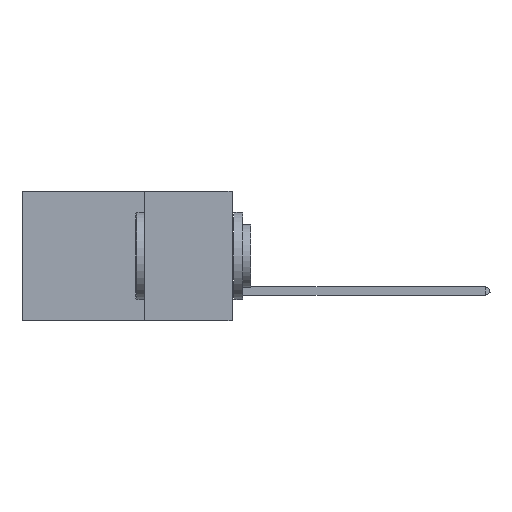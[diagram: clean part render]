
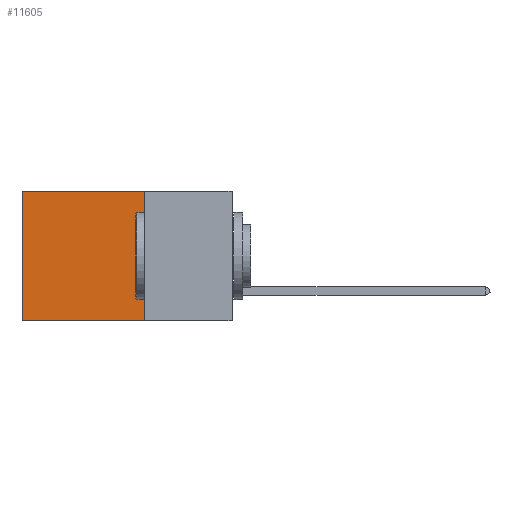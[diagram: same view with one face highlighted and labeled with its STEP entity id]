
A CAD part, left-side view. The second image highlights one B-rep face of the part: STEP entity #11605.
In plain terms, the highlighted planar face has unit normal (-1, 0, 0).
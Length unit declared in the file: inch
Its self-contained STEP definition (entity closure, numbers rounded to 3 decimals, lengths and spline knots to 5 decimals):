
#1094 = DIRECTION ( 'NONE',  ( 0., 1., 0. ) ) ;
#1819 = EDGE_CURVE ( 'NONE', #19854, #14583, #12272, .T. ) ;
#1836 = CARTESIAN_POINT ( 'NONE',  ( 0.2875, 0.25, 0. ) ) ;
#2505 = CARTESIAN_POINT ( 'NONE',  ( 0.2875, 0.25, -0.37 ) ) ;
#5303 = VECTOR ( 'NONE', #8890, 39.37008 ) ;
#5364 = EDGE_CURVE ( 'NONE', #10749, #14583, #9433, .T. ) ;
#5891 = ORIENTED_EDGE ( 'NONE', *, *, #1819, .F. ) ;
#6090 = VERTEX_POINT ( 'NONE', #13064 ) ;
#6098 = LINE ( 'NONE', #1836, #5303 ) ;
#7207 = FACE_OUTER_BOUND ( 'NONE', #11936, .T. ) ;
#8653 = ORIENTED_EDGE ( 'NONE', *, *, #5364, .T. ) ;
#8890 = DIRECTION ( 'NONE',  ( 0., 0., -1. ) ) ;
#9433 = LINE ( 'NONE', #11645, #18881 ) ;
#10124 = VECTOR ( 'NONE', #1094, 39.37008 ) ;
#10749 = VERTEX_POINT ( 'NONE', #15766 ) ;
#11398 = CARTESIAN_POINT ( 'NONE',  ( 0.2875, 0.25, -0.37 ) ) ;
#11605 = ADVANCED_FACE ( 'NONE', ( #7207 ), #14404, .F. ) ;
#11645 = CARTESIAN_POINT ( 'NONE',  ( 0.2875, 0.6, 0. ) ) ;
#11936 = EDGE_LOOP ( 'NONE', ( #8653, #5891, #16373, #12338 ) ) ;
#12272 = LINE ( 'NONE', #11398, #10124 ) ;
#12328 = VECTOR ( 'NONE', #18342, 39.37008 ) ;
#12338 = ORIENTED_EDGE ( 'NONE', *, *, #15998, .T. ) ;
#12956 = DIRECTION ( 'NONE',  ( 0., 0., -1. ) ) ;
#13064 = CARTESIAN_POINT ( 'NONE',  ( 0.2875, 0.25, 0. ) ) ;
#13457 = CARTESIAN_POINT ( 'NONE',  ( 0.2875, 0.25, 0. ) ) ;
#14404 = PLANE ( 'NONE',  #16626 ) ;
#14583 = VERTEX_POINT ( 'NONE', #17863 ) ;
#15766 = CARTESIAN_POINT ( 'NONE',  ( 0.2875, 0.6, 0. ) ) ;
#15998 = EDGE_CURVE ( 'NONE', #6090, #10749, #19354, .T. ) ;
#16349 = EDGE_CURVE ( 'NONE', #6090, #19854, #6098, .T. ) ;
#16373 = ORIENTED_EDGE ( 'NONE', *, *, #16349, .F. ) ;
#16626 = AXIS2_PLACEMENT_3D ( 'NONE', #13457, #16948, #12956 ) ;
#16948 = DIRECTION ( 'NONE',  ( 1., 0., 0. ) ) ;
#17863 = CARTESIAN_POINT ( 'NONE',  ( 0.2875, 0.6, -0.37 ) ) ;
#18192 = CARTESIAN_POINT ( 'NONE',  ( 0.2875, 0.25, 0. ) ) ;
#18342 = DIRECTION ( 'NONE',  ( 0., 1., 0. ) ) ;
#18881 = VECTOR ( 'NONE', #19328, 39.37008 ) ;
#19328 = DIRECTION ( 'NONE',  ( 0., 0., -1. ) ) ;
#19354 = LINE ( 'NONE', #18192, #12328 ) ;
#19854 = VERTEX_POINT ( 'NONE', #2505 ) ;
